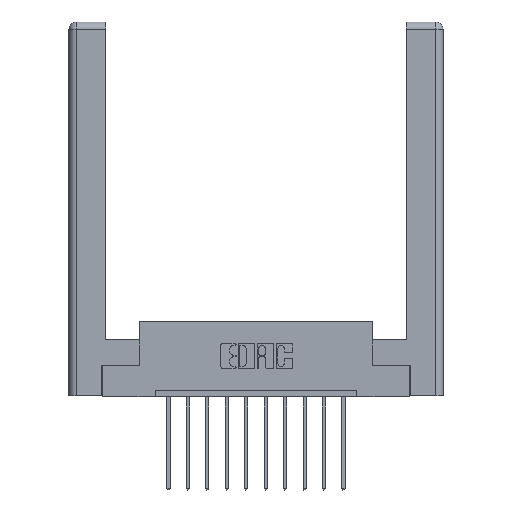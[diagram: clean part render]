
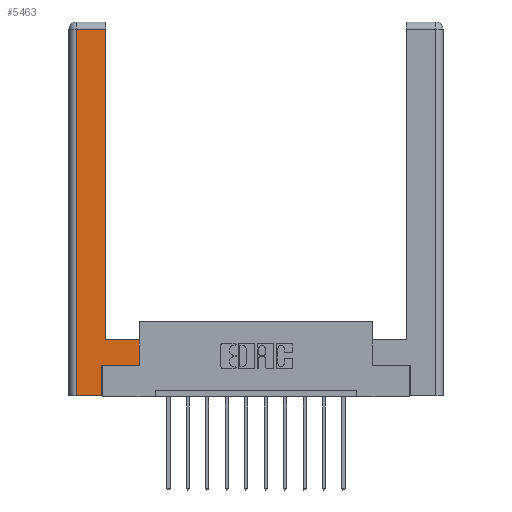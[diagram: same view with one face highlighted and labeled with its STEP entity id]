
A CAD part, top view. The second image highlights one B-rep face of the part: STEP entity #5463.
In plain terms, the highlighted planar face has unit normal (0, 0, 1).
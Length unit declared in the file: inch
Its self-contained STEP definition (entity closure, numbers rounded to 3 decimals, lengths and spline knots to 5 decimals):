
#18 = ORIENTED_EDGE ( 'NONE', *, *, #6865, .T. ) ;
#58 = VECTOR ( 'NONE', #1840, 39.37008 ) ;
#61 = DIRECTION ( 'NONE',  ( -1., 0., 0. ) ) ;
#122 = VECTOR ( 'NONE', #1463, 39.37008 ) ;
#314 = ORIENTED_EDGE ( 'NONE', *, *, #9705, .T. ) ;
#951 = DIRECTION ( 'NONE',  ( 0., -1., 0. ) ) ;
#1009 = CARTESIAN_POINT ( 'NONE',  ( 0., 0., 0. ) ) ;
#1234 = VERTEX_POINT ( 'NONE', #11676 ) ;
#1463 = DIRECTION ( 'NONE',  ( 0., 1., 0. ) ) ;
#1798 = CARTESIAN_POINT ( 'NONE',  ( 0.0615, 0., 0. ) ) ;
#1840 = DIRECTION ( 'NONE',  ( 1., 0., 0. ) ) ;
#2031 = VECTOR ( 'NONE', #5693, 39.37008 ) ;
#2158 = PLANE ( 'NONE',  #11703 ) ;
#2355 = EDGE_CURVE ( 'NONE', #8806, #5725, #5802, .T. ) ;
#2372 = ORIENTED_EDGE ( 'NONE', *, *, #3886, .T. ) ;
#2425 = VECTOR ( 'NONE', #8813, 39.37008 ) ;
#2664 = CARTESIAN_POINT ( 'NONE',  ( 0.295, 0.45, 0. ) ) ;
#2671 = CARTESIAN_POINT ( 'NONE',  ( 0.265, 0., 0. ) ) ;
#2752 = DIRECTION ( 'NONE',  ( -1., 0., 0. ) ) ;
#2931 = CARTESIAN_POINT ( 'NONE',  ( 0.295, 3., 0. ) ) ;
#3083 = ORIENTED_EDGE ( 'NONE', *, *, #5662, .T. ) ;
#3221 = VECTOR ( 'NONE', #3448, 39.37008 ) ;
#3418 = LINE ( 'NONE', #4479, #2031 ) ;
#3448 = DIRECTION ( 'NONE',  ( -1., 0., 0. ) ) ;
#3482 = CARTESIAN_POINT ( 'NONE',  ( 0.295, 2.94, 0. ) ) ;
#3886 = EDGE_CURVE ( 'NONE', #5725, #11911, #12049, .T. ) ;
#3923 = VERTEX_POINT ( 'NONE', #1798 ) ;
#3959 = VERTEX_POINT ( 'NONE', #3482 ) ;
#4021 = EDGE_LOOP ( 'NONE', ( #3083, #5313, #314, #4823, #10801, #2372, #18, #6165 ) ) ;
#4312 = FACE_OUTER_BOUND ( 'NONE', #4021, .T. ) ;
#4479 = CARTESIAN_POINT ( 'NONE',  ( 0.265, 0., 0. ) ) ;
#4823 = ORIENTED_EDGE ( 'NONE', *, *, #6257, .T. ) ;
#4900 = EDGE_CURVE ( 'NONE', #3959, #7687, #8258, .T. ) ;
#5313 = ORIENTED_EDGE ( 'NONE', *, *, #4900, .T. ) ;
#5463 = ADVANCED_FACE ( 'NONE', ( #4312 ), #2158, .F. ) ;
#5662 = EDGE_CURVE ( 'NONE', #13256, #3959, #8407, .T. ) ;
#5693 = DIRECTION ( 'NONE',  ( 1., 0., 0. ) ) ;
#5725 = VERTEX_POINT ( 'NONE', #11967 ) ;
#5802 = LINE ( 'NONE', #9901, #2425 ) ;
#6156 = LINE ( 'NONE', #10013, #3221 ) ;
#6165 = ORIENTED_EDGE ( 'NONE', *, *, #6819, .T. ) ;
#6257 = EDGE_CURVE ( 'NONE', #3923, #8806, #3418, .T. ) ;
#6819 = EDGE_CURVE ( 'NONE', #1234, #13256, #6156, .T. ) ;
#6865 = EDGE_CURVE ( 'NONE', #11911, #1234, #8882, .T. ) ;
#6873 = VECTOR ( 'NONE', #2752, 39.37008 ) ;
#7028 = VECTOR ( 'NONE', #7361, 39.37008 ) ;
#7361 = DIRECTION ( 'NONE',  ( 0., 1., 0. ) ) ;
#7519 = CARTESIAN_POINT ( 'NONE',  ( 0.0615, 0., 0. ) ) ;
#7687 = VERTEX_POINT ( 'NONE', #8874 ) ;
#8258 = LINE ( 'NONE', #13727, #6873 ) ;
#8407 = LINE ( 'NONE', #2931, #7028 ) ;
#8806 = VERTEX_POINT ( 'NONE', #2671 ) ;
#8813 = DIRECTION ( 'NONE',  ( 0., 1., 0. ) ) ;
#8874 = CARTESIAN_POINT ( 'NONE',  ( 0.0615, 2.94, 0. ) ) ;
#8882 = LINE ( 'NONE', #12491, #122 ) ;
#9438 = CARTESIAN_POINT ( 'NONE',  ( 0.565, 0.245, 0. ) ) ;
#9705 = EDGE_CURVE ( 'NONE', #7687, #3923, #10010, .T. ) ;
#9901 = CARTESIAN_POINT ( 'NONE',  ( 0.265, 0.245, 0. ) ) ;
#10010 = LINE ( 'NONE', #7519, #13086 ) ;
#10013 = CARTESIAN_POINT ( 'NONE',  ( 0.295, 0.45, 0. ) ) ;
#10801 = ORIENTED_EDGE ( 'NONE', *, *, #2355, .T. ) ;
#11676 = CARTESIAN_POINT ( 'NONE',  ( 0.565, 0.45, 0. ) ) ;
#11703 = AXIS2_PLACEMENT_3D ( 'NONE', #1009, #14176, #61 ) ;
#11911 = VERTEX_POINT ( 'NONE', #13539 ) ;
#11967 = CARTESIAN_POINT ( 'NONE',  ( 0.265, 0.245, 0. ) ) ;
#12049 = LINE ( 'NONE', #9438, #58 ) ;
#12491 = CARTESIAN_POINT ( 'NONE',  ( 0.565, 0.45, 0. ) ) ;
#13086 = VECTOR ( 'NONE', #951, 39.37008 ) ;
#13256 = VERTEX_POINT ( 'NONE', #2664 ) ;
#13539 = CARTESIAN_POINT ( 'NONE',  ( 0.565, 0.245, 0. ) ) ;
#13727 = CARTESIAN_POINT ( 'NONE',  ( 0.0615, 2.94, 0. ) ) ;
#14176 = DIRECTION ( 'NONE',  ( 0., 0., -1. ) ) ;
